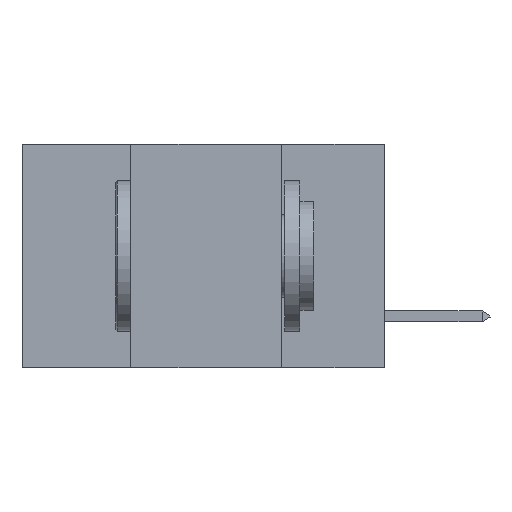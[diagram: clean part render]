
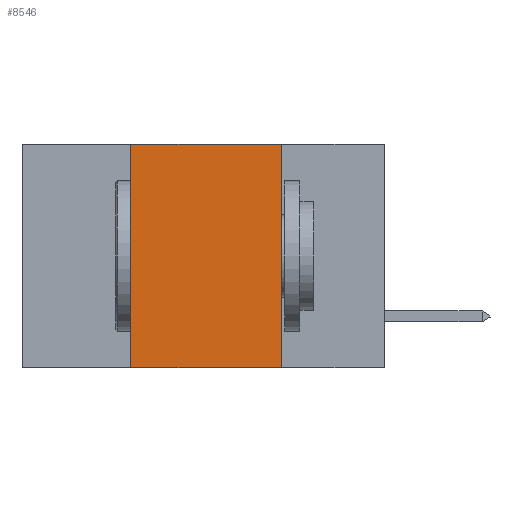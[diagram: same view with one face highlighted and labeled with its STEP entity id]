
A CAD part, left-side view. The second image highlights one B-rep face of the part: STEP entity #8546.
In plain terms, the highlighted planar face has unit normal (-1, 0, 0).
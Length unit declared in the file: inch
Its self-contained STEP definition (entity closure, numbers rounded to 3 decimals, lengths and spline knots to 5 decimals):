
#102 = CARTESIAN_POINT ( 'NONE',  ( 0., 0.17, -0.37 ) ) ;
#671 = CARTESIAN_POINT ( 'NONE',  ( 0., 0.42, -0.37 ) ) ;
#828 = VECTOR ( 'NONE', #3392, 39.37008 ) ;
#1478 = VECTOR ( 'NONE', #4777, 39.37008 ) ;
#1536 = VERTEX_POINT ( 'NONE', #8097 ) ;
#2003 = VECTOR ( 'NONE', #2476, 39.37008 ) ;
#2476 = DIRECTION ( 'NONE',  ( 0., -1., 0. ) ) ;
#2502 = CARTESIAN_POINT ( 'NONE',  ( 0., 0.17, 0. ) ) ;
#2780 = EDGE_CURVE ( 'NONE', #3932, #16395, #10425, .T. ) ;
#3290 = CARTESIAN_POINT ( 'NONE',  ( 0., 0.6, -0.37 ) ) ;
#3392 = DIRECTION ( 'NONE',  ( 0., 0., 1. ) ) ;
#3932 = VERTEX_POINT ( 'NONE', #671 ) ;
#4777 = DIRECTION ( 'NONE',  ( 0., 0., -1. ) ) ;
#4939 = FACE_OUTER_BOUND ( 'NONE', #10522, .T. ) ;
#5108 = ORIENTED_EDGE ( 'NONE', *, *, #15627, .F. ) ;
#5888 = LINE ( 'NONE', #9446, #14364 ) ;
#6708 = ORIENTED_EDGE ( 'NONE', *, *, #11474, .F. ) ;
#7627 = LINE ( 'NONE', #16662, #1478 ) ;
#7629 = DIRECTION ( 'NONE',  ( 0., 0., -1. ) ) ;
#7798 = LINE ( 'NONE', #11321, #828 ) ;
#8075 = EDGE_CURVE ( 'NONE', #14429, #16395, #7627, .T. ) ;
#8097 = CARTESIAN_POINT ( 'NONE',  ( 0., 0.42, 0. ) ) ;
#8546 = ADVANCED_FACE ( 'NONE', ( #4939 ), #14179, .F. ) ;
#8888 = CARTESIAN_POINT ( 'NONE',  ( 0., 0.6, 0. ) ) ;
#9446 = CARTESIAN_POINT ( 'NONE',  ( 0., 0.6, 0. ) ) ;
#10425 = LINE ( 'NONE', #3290, #2003 ) ;
#10522 = EDGE_LOOP ( 'NONE', ( #11904, #6708, #5108, #16300 ) ) ;
#10943 = AXIS2_PLACEMENT_3D ( 'NONE', #8888, #16763, #7629 ) ;
#11321 = CARTESIAN_POINT ( 'NONE',  ( 0., 0.42, 0. ) ) ;
#11474 = EDGE_CURVE ( 'NONE', #1536, #14429, #5888, .T. ) ;
#11904 = ORIENTED_EDGE ( 'NONE', *, *, #8075, .F. ) ;
#14179 = PLANE ( 'NONE',  #10943 ) ;
#14364 = VECTOR ( 'NONE', #14676, 39.37008 ) ;
#14429 = VERTEX_POINT ( 'NONE', #2502 ) ;
#14676 = DIRECTION ( 'NONE',  ( 0., -1., 0. ) ) ;
#15627 = EDGE_CURVE ( 'NONE', #3932, #1536, #7798, .T. ) ;
#16300 = ORIENTED_EDGE ( 'NONE', *, *, #2780, .T. ) ;
#16395 = VERTEX_POINT ( 'NONE', #102 ) ;
#16662 = CARTESIAN_POINT ( 'NONE',  ( 0., 0.17, 0. ) ) ;
#16763 = DIRECTION ( 'NONE',  ( 1., 0., 0. ) ) ;
